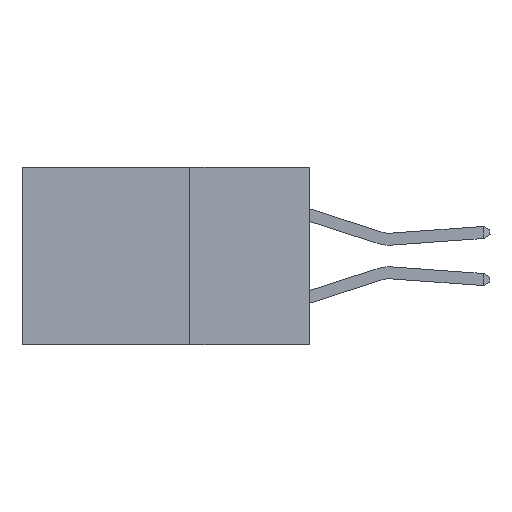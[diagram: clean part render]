
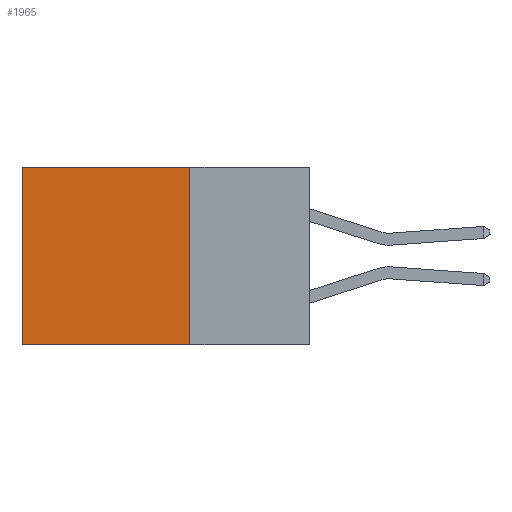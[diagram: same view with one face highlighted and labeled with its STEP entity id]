
A CAD part, left-side view. The second image highlights one B-rep face of the part: STEP entity #1965.
In plain terms, the highlighted planar face has unit normal (-1, 0, 0).
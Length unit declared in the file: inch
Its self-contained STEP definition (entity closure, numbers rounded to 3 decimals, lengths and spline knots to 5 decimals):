
#169 = ORIENTED_EDGE ( 'NONE', *, *, #2082, .T. ) ;
#622 = ORIENTED_EDGE ( 'NONE', *, *, #9555, .F. ) ;
#660 = DIRECTION ( 'NONE',  ( 0., 0., -1. ) ) ;
#723 = VECTOR ( 'NONE', #7127, 39.37008 ) ;
#850 = VERTEX_POINT ( 'NONE', #11063 ) ;
#900 = CARTESIAN_POINT ( 'NONE',  ( 0.2615, 0.25, -0.37 ) ) ;
#1965 = ADVANCED_FACE ( 'NONE', ( #14980 ), #11076, .F. ) ;
#2082 = EDGE_CURVE ( 'NONE', #14815, #8248, #4060, .T. ) ;
#2109 = LINE ( 'NONE', #900, #11493 ) ;
#3542 = LINE ( 'NONE', #14742, #12471 ) ;
#3580 = VERTEX_POINT ( 'NONE', #4680 ) ;
#3832 = CARTESIAN_POINT ( 'NONE',  ( 0.2615, 0.6, -0.37 ) ) ;
#4060 = LINE ( 'NONE', #7453, #723 ) ;
#4680 = CARTESIAN_POINT ( 'NONE',  ( 0.2615, 0.25, -0.37 ) ) ;
#4769 = LINE ( 'NONE', #13727, #14227 ) ;
#6078 = AXIS2_PLACEMENT_3D ( 'NONE', #10793, #10190, #10168 ) ;
#6661 = CARTESIAN_POINT ( 'NONE',  ( 0.2615, 0.6, 0. ) ) ;
#6967 = ORIENTED_EDGE ( 'NONE', *, *, #9885, .T. ) ;
#7127 = DIRECTION ( 'NONE',  ( 0., 0., -1. ) ) ;
#7453 = CARTESIAN_POINT ( 'NONE',  ( 0.2615, 0.6, -0.37 ) ) ;
#8248 = VERTEX_POINT ( 'NONE', #3832 ) ;
#9555 = EDGE_CURVE ( 'NONE', #850, #3580, #2109, .T. ) ;
#9885 = EDGE_CURVE ( 'NONE', #850, #14815, #4769, .T. ) ;
#10029 = EDGE_CURVE ( 'NONE', #3580, #8248, #3542, .T. ) ;
#10168 = DIRECTION ( 'NONE',  ( 0., 0., -1. ) ) ;
#10190 = DIRECTION ( 'NONE',  ( 1., 0., 0. ) ) ;
#10793 = CARTESIAN_POINT ( 'NONE',  ( 0.2615, 0.25, -0.37 ) ) ;
#11063 = CARTESIAN_POINT ( 'NONE',  ( 0.2615, 0.25, 0. ) ) ;
#11076 = PLANE ( 'NONE',  #6078 ) ;
#11493 = VECTOR ( 'NONE', #660, 39.37008 ) ;
#12471 = VECTOR ( 'NONE', #14688, 39.37008 ) ;
#13678 = DIRECTION ( 'NONE',  ( 0., 1., 0. ) ) ;
#13685 = EDGE_LOOP ( 'NONE', ( #169, #14428, #622, #6967 ) ) ;
#13727 = CARTESIAN_POINT ( 'NONE',  ( 0.2615, 0.25, 0. ) ) ;
#14227 = VECTOR ( 'NONE', #13678, 39.37008 ) ;
#14428 = ORIENTED_EDGE ( 'NONE', *, *, #10029, .F. ) ;
#14688 = DIRECTION ( 'NONE',  ( 0., 1., 0. ) ) ;
#14742 = CARTESIAN_POINT ( 'NONE',  ( 0.2615, 0.25, -0.37 ) ) ;
#14815 = VERTEX_POINT ( 'NONE', #6661 ) ;
#14980 = FACE_OUTER_BOUND ( 'NONE', #13685, .T. ) ;
